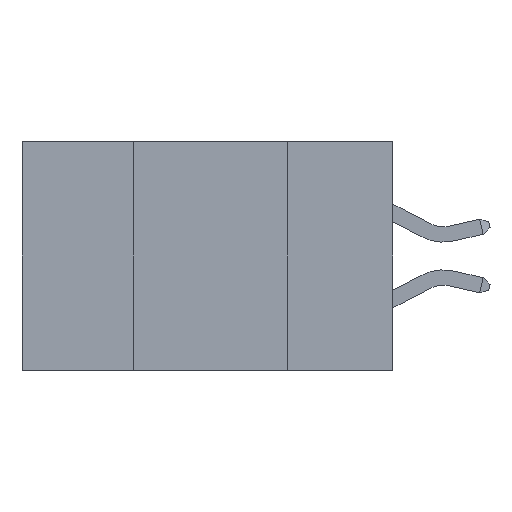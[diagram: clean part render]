
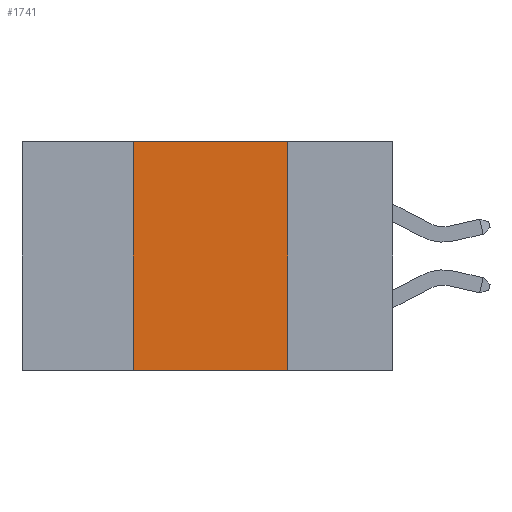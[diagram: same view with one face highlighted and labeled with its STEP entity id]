
A CAD part, left-side view. The second image highlights one B-rep face of the part: STEP entity #1741.
In plain terms, the highlighted planar face has unit normal (-1, 0, 0).
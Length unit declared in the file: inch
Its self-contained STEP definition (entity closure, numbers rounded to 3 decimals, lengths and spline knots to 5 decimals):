
#1314 = EDGE_CURVE ( 'NONE', #3452, #14503, #1481, .T. ) ;
#1481 = LINE ( 'NONE', #12253, #2709 ) ;
#1741 = ADVANCED_FACE ( 'NONE', ( #5402 ), #2744, .F. ) ;
#2057 = EDGE_CURVE ( 'NONE', #10884, #3452, #4220, .T. ) ;
#2289 = DIRECTION ( 'NONE',  ( 0., -1., 0. ) ) ;
#2405 = DIRECTION ( 'NONE',  ( 0., 0., -1. ) ) ;
#2709 = VECTOR ( 'NONE', #13422, 39.37008 ) ;
#2744 = PLANE ( 'NONE',  #11325 ) ;
#3452 = VERTEX_POINT ( 'NONE', #15624 ) ;
#4220 = LINE ( 'NONE', #4563, #5646 ) ;
#4419 = LINE ( 'NONE', #7494, #15695 ) ;
#4563 = CARTESIAN_POINT ( 'NONE',  ( 0., 0.42, 0. ) ) ;
#5402 = FACE_OUTER_BOUND ( 'NONE', #9913, .T. ) ;
#5646 = VECTOR ( 'NONE', #11027, 39.37008 ) ;
#6102 = ORIENTED_EDGE ( 'NONE', *, *, #9930, .T. ) ;
#6879 = CARTESIAN_POINT ( 'NONE',  ( 0., 0.17, 0. ) ) ;
#7494 = CARTESIAN_POINT ( 'NONE',  ( 0., 0.6, -0.37 ) ) ;
#7676 = VECTOR ( 'NONE', #2405, 39.37008 ) ;
#7751 = CARTESIAN_POINT ( 'NONE',  ( 0., 0.17, -0.37 ) ) ;
#7783 = CARTESIAN_POINT ( 'NONE',  ( 0., 0.17, 0. ) ) ;
#7956 = ORIENTED_EDGE ( 'NONE', *, *, #2057, .F. ) ;
#8221 = CARTESIAN_POINT ( 'NONE',  ( 0., 0.42, -0.37 ) ) ;
#8601 = ORIENTED_EDGE ( 'NONE', *, *, #1314, .F. ) ;
#8814 = CARTESIAN_POINT ( 'NONE',  ( 0., 0.6, 0. ) ) ;
#9363 = VERTEX_POINT ( 'NONE', #7751 ) ;
#9913 = EDGE_LOOP ( 'NONE', ( #15899, #8601, #7956, #6102 ) ) ;
#9930 = EDGE_CURVE ( 'NONE', #10884, #9363, #4419, .T. ) ;
#10564 = LINE ( 'NONE', #7783, #7676 ) ;
#10884 = VERTEX_POINT ( 'NONE', #8221 ) ;
#11027 = DIRECTION ( 'NONE',  ( 0., 0., 1. ) ) ;
#11325 = AXIS2_PLACEMENT_3D ( 'NONE', #8814, #15435, #15873 ) ;
#12253 = CARTESIAN_POINT ( 'NONE',  ( 0., 0.6, 0. ) ) ;
#13422 = DIRECTION ( 'NONE',  ( 0., -1., 0. ) ) ;
#14503 = VERTEX_POINT ( 'NONE', #6879 ) ;
#15435 = DIRECTION ( 'NONE',  ( 1., 0., 0. ) ) ;
#15624 = CARTESIAN_POINT ( 'NONE',  ( 0., 0.42, 0. ) ) ;
#15695 = VECTOR ( 'NONE', #2289, 39.37008 ) ;
#15873 = DIRECTION ( 'NONE',  ( 0., 0., -1. ) ) ;
#15899 = ORIENTED_EDGE ( 'NONE', *, *, #16261, .F. ) ;
#16261 = EDGE_CURVE ( 'NONE', #14503, #9363, #10564, .T. ) ;
